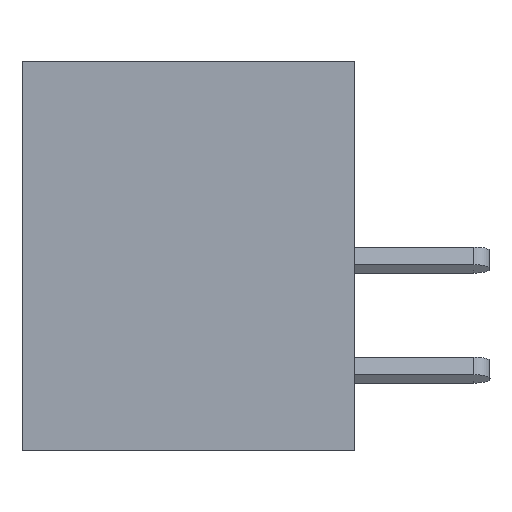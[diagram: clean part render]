
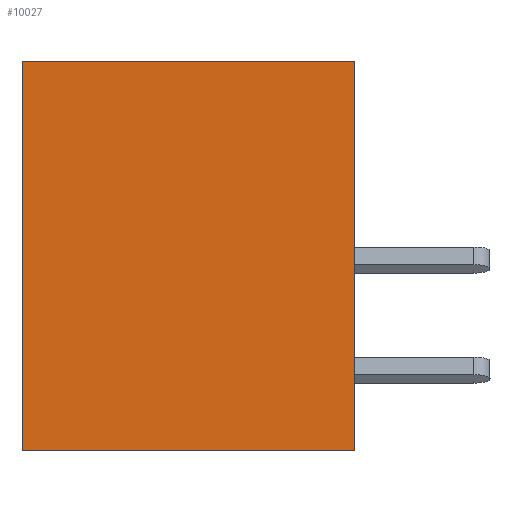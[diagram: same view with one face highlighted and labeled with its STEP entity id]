
A CAD part, left-side view. The second image highlights one B-rep face of the part: STEP entity #10027.
In plain terms, the highlighted planar face has unit normal (-1, 0, 0).
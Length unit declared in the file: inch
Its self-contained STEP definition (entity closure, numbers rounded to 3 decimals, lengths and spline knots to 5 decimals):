
#551 = DIRECTION ( 'NONE',  ( 0., 0., 1. ) ) ;
#1438 = FACE_OUTER_BOUND ( 'NONE', #28203, .T. ) ;
#1910 = VECTOR ( 'NONE', #12433, 39.37008 ) ;
#1947 = CARTESIAN_POINT ( 'NONE',  ( 0., 0.453, 0. ) ) ;
#3207 = CARTESIAN_POINT ( 'NONE',  ( 0., 0., 0. ) ) ;
#3308 = DIRECTION ( 'NONE',  ( 0., 0., 1. ) ) ;
#3748 = CARTESIAN_POINT ( 'NONE',  ( 0., 0.453, -0.531 ) ) ;
#4334 = LINE ( 'NONE', #10412, #1910 ) ;
#5502 = CARTESIAN_POINT ( 'NONE',  ( 0., 0., -0.531 ) ) ;
#6315 = DIRECTION ( 'NONE',  ( 1., 0., 0. ) ) ;
#7348 = DIRECTION ( 'NONE',  ( 0., -1., 0. ) ) ;
#7470 = VECTOR ( 'NONE', #551, 39.37008 ) ;
#7934 = VERTEX_POINT ( 'NONE', #9757 ) ;
#8959 = DIRECTION ( 'NONE',  ( 0., 0., -1. ) ) ;
#9751 = EDGE_CURVE ( 'NONE', #21902, #7934, #17055, .T. ) ;
#9757 = CARTESIAN_POINT ( 'NONE',  ( 0., 0., 0. ) ) ;
#10027 = ADVANCED_FACE ( 'NONE', ( #1438 ), #17171, .F. ) ;
#10412 = CARTESIAN_POINT ( 'NONE',  ( 0., 0.453, 0. ) ) ;
#12433 = DIRECTION ( 'NONE',  ( 0., -1., 0. ) ) ;
#13652 = EDGE_CURVE ( 'NONE', #23841, #23605, #19220, .T. ) ;
#14111 = CARTESIAN_POINT ( 'NONE',  ( 0., 0.453, -0.531 ) ) ;
#14298 = EDGE_CURVE ( 'NONE', #23841, #21902, #26520, .T. ) ;
#14977 = VECTOR ( 'NONE', #3308, 39.37008 ) ;
#15675 = EDGE_CURVE ( 'NONE', #23605, #7934, #4334, .T. ) ;
#16468 = CARTESIAN_POINT ( 'NONE',  ( 0., 0.453, 0. ) ) ;
#17055 = LINE ( 'NONE', #3207, #14977 ) ;
#17171 = PLANE ( 'NONE',  #18982 ) ;
#18982 = AXIS2_PLACEMENT_3D ( 'NONE', #1947, #6315, #8959 ) ;
#19220 = LINE ( 'NONE', #16468, #7470 ) ;
#19428 = ORIENTED_EDGE ( 'NONE', *, *, #13652, .F. ) ;
#20615 = VECTOR ( 'NONE', #7348, 39.37008 ) ;
#21902 = VERTEX_POINT ( 'NONE', #5502 ) ;
#21955 = ORIENTED_EDGE ( 'NONE', *, *, #14298, .T. ) ;
#23605 = VERTEX_POINT ( 'NONE', #27159 ) ;
#23841 = VERTEX_POINT ( 'NONE', #3748 ) ;
#25401 = ORIENTED_EDGE ( 'NONE', *, *, #15675, .F. ) ;
#26520 = LINE ( 'NONE', #14111, #20615 ) ;
#27159 = CARTESIAN_POINT ( 'NONE',  ( 0., 0.453, 0. ) ) ;
#27458 = ORIENTED_EDGE ( 'NONE', *, *, #9751, .T. ) ;
#28203 = EDGE_LOOP ( 'NONE', ( #27458, #25401, #19428, #21955 ) ) ;
